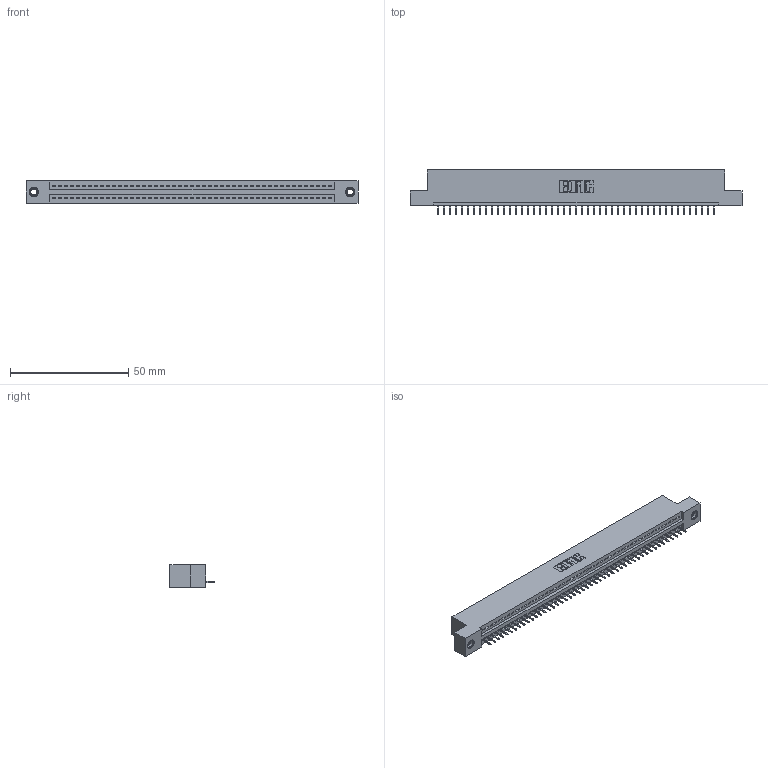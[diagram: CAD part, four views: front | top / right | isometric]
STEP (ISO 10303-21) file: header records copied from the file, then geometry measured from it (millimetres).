
FILE_DESCRIPTION (( 'STEP AP203' ), '1' );
FILE_NAME ('345-047-525-107.STEP', '2020-09-20T00:24:53', ( '' ), ( '' ), 'SwSTEP 2.0', 'SolidWorks 2020', '' );
FILE_SCHEMA (( 'CONFIG_CONTROL_DESIGN' ));
Length unit declared in the file: inch
Products named in the file (4): 345-292-001_345-293-125; 345 Part_Flush Mounting Lugs - 0.156 Dia-TI; 345-250-001_345-250-005-103; 345-047-525-107
Assembly tree (50 placements, depth 2):
  345-047-525-107
    345 Part_Flush Mounting Lugs - 0.156 Dia-TI
    345-292-001_345-293-125  x47
    345-250-001_345-250-005-103  x2
Bounding box: 140.59 x 18.72 x 9.4 mm (x, y, z)
Volume: 13188.8 mm3; surface area: 16987.3 mm2
Topology: 50 solids, 50 shells, 3100 faces, 8937 edges, 5762 vertices
Faces by surface type: plane 2274, cylinder 810, cone 12, torus 4
Entity records: 35960 total; most frequent: CARTESIAN_POINT 6208, ORIENTED_EDGE 6182, DIRECTION 5443, EDGE_CURVE 3091, VECTOR 2755, LINE 2755, VERTEX_POINT 2052, AXIS2_PLACEMENT_3D 1344
